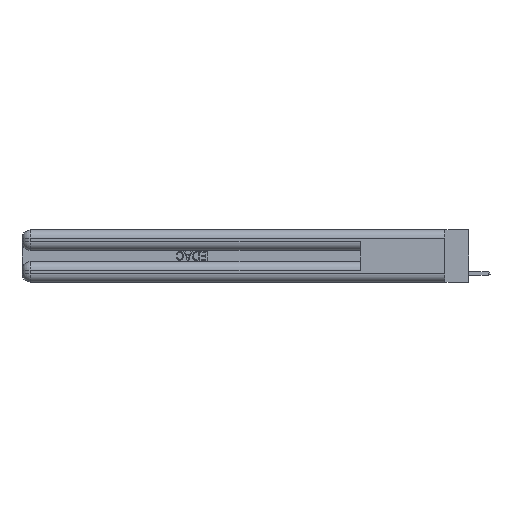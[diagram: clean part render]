
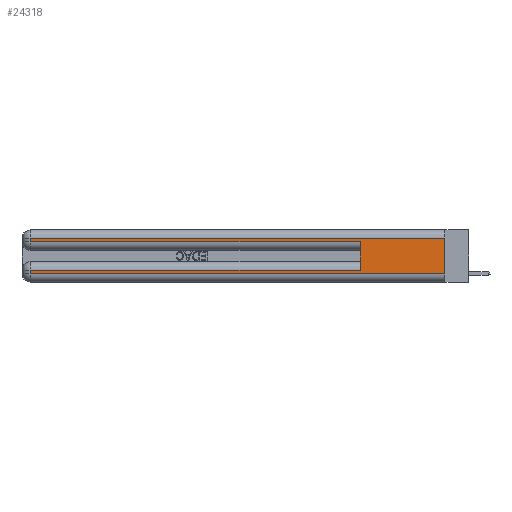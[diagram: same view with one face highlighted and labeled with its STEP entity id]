
A CAD part, left-side view. The second image highlights one B-rep face of the part: STEP entity #24318.
In plain terms, the highlighted planar face has unit normal (-1, 0, 0).
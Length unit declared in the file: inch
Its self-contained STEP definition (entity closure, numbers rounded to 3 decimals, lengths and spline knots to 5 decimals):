
#934 = DIRECTION ( 'NONE',  ( 0., 1., 0. ) ) ;
#1183 = DIRECTION ( 'NONE',  ( 0., -1., 0. ) ) ;
#1194 = VECTOR ( 'NONE', #3811, 39.37008 ) ;
#1406 = EDGE_LOOP ( 'NONE', ( #26395, #14939, #14035, #9605, #3924, #25589, #17612, #13681 ) ) ;
#1484 = EDGE_CURVE ( 'NONE', #33458, #34195, #20862, .T. ) ;
#1713 = VERTEX_POINT ( 'NONE', #23563 ) ;
#1804 = EDGE_CURVE ( 'NONE', #1713, #3582, #31366, .T. ) ;
#3386 = DIRECTION ( 'NONE',  ( 0., 0., -1. ) ) ;
#3582 = VERTEX_POINT ( 'NONE', #27402 ) ;
#3811 = DIRECTION ( 'NONE',  ( 0., 0., -1. ) ) ;
#3924 = ORIENTED_EDGE ( 'NONE', *, *, #13835, .F. ) ;
#4357 = CARTESIAN_POINT ( 'NONE',  ( 0., 2.94, 0.31 ) ) ;
#4922 = LINE ( 'NONE', #22695, #1194 ) ;
#5333 = VECTOR ( 'NONE', #3386, 39.37008 ) ;
#5536 = CARTESIAN_POINT ( 'NONE',  ( 0., 0.6, 0.145 ) ) ;
#5852 = CARTESIAN_POINT ( 'NONE',  ( 0., 0., 0.06 ) ) ;
#8537 = LINE ( 'NONE', #18350, #33734 ) ;
#8920 = CARTESIAN_POINT ( 'NONE',  ( 0., 0., 0.285 ) ) ;
#9605 = ORIENTED_EDGE ( 'NONE', *, *, #1484, .T. ) ;
#11579 = EDGE_CURVE ( 'NONE', #33373, #33458, #32306, .T. ) ;
#13681 = ORIENTED_EDGE ( 'NONE', *, *, #33790, .T. ) ;
#13835 = EDGE_CURVE ( 'NONE', #33293, #34195, #23214, .T. ) ;
#14035 = ORIENTED_EDGE ( 'NONE', *, *, #11579, .T. ) ;
#14939 = ORIENTED_EDGE ( 'NONE', *, *, #26741, .T. ) ;
#15154 = DIRECTION ( 'NONE',  ( 0., 1., 0. ) ) ;
#15432 = VECTOR ( 'NONE', #934, 39.37008 ) ;
#15842 = VECTOR ( 'NONE', #18857, 39.37008 ) ;
#16941 = CARTESIAN_POINT ( 'NONE',  ( 0., 2.94, 0.37 ) ) ;
#16946 = EDGE_CURVE ( 'NONE', #29055, #30956, #4922, .T. ) ;
#17269 = DIRECTION ( 'NONE',  ( 1., 0., 0. ) ) ;
#17492 = VECTOR ( 'NONE', #1183, 39.37008 ) ;
#17612 = ORIENTED_EDGE ( 'NONE', *, *, #1804, .T. ) ;
#18350 = CARTESIAN_POINT ( 'NONE',  ( 0., 0., 0.06 ) ) ;
#18857 = DIRECTION ( 'NONE',  ( 0., 0., -1. ) ) ;
#20640 = CARTESIAN_POINT ( 'NONE',  ( 0., 0.6, 0.085 ) ) ;
#20862 = LINE ( 'NONE', #8920, #17492 ) ;
#21330 = CARTESIAN_POINT ( 'NONE',  ( 0., 2.94, 0.37 ) ) ;
#22695 = CARTESIAN_POINT ( 'NONE',  ( 0., 0., 0.37 ) ) ;
#23214 = LINE ( 'NONE', #5536, #26163 ) ;
#23563 = CARTESIAN_POINT ( 'NONE',  ( 0., 2.94, 0.085 ) ) ;
#23775 = DIRECTION ( 'NONE',  ( 0., -1., 0. ) ) ;
#24248 = LINE ( 'NONE', #33930, #34741 ) ;
#24318 = ADVANCED_FACE ( 'NONE', ( #31562 ), #27409, .F. ) ;
#25128 = CARTESIAN_POINT ( 'NONE',  ( 0., 0., 0.085 ) ) ;
#25542 = DIRECTION ( 'NONE',  ( 0., 0., -1. ) ) ;
#25589 = ORIENTED_EDGE ( 'NONE', *, *, #26353, .T. ) ;
#26163 = VECTOR ( 'NONE', #32309, 39.37008 ) ;
#26353 = EDGE_CURVE ( 'NONE', #33293, #1713, #28062, .T. ) ;
#26395 = ORIENTED_EDGE ( 'NONE', *, *, #16946, .F. ) ;
#26723 = CARTESIAN_POINT ( 'NONE',  ( 0., 0., 0.31 ) ) ;
#26741 = EDGE_CURVE ( 'NONE', #29055, #33373, #24248, .T. ) ;
#27402 = CARTESIAN_POINT ( 'NONE',  ( 0., 2.94, 0.06 ) ) ;
#27409 = PLANE ( 'NONE',  #30368 ) ;
#28062 = LINE ( 'NONE', #25128, #15432 ) ;
#29055 = VERTEX_POINT ( 'NONE', #26723 ) ;
#30368 = AXIS2_PLACEMENT_3D ( 'NONE', #32815, #17269, #25542 ) ;
#30956 = VERTEX_POINT ( 'NONE', #5852 ) ;
#31366 = LINE ( 'NONE', #16941, #5333 ) ;
#31562 = FACE_OUTER_BOUND ( 'NONE', #1406, .T. ) ;
#32306 = LINE ( 'NONE', #21330, #15842 ) ;
#32309 = DIRECTION ( 'NONE',  ( 0., 0., 1. ) ) ;
#32815 = CARTESIAN_POINT ( 'NONE',  ( 0., 0., 0.37 ) ) ;
#33293 = VERTEX_POINT ( 'NONE', #20640 ) ;
#33373 = VERTEX_POINT ( 'NONE', #4357 ) ;
#33390 = CARTESIAN_POINT ( 'NONE',  ( 0., 0.6, 0.285 ) ) ;
#33458 = VERTEX_POINT ( 'NONE', #34629 ) ;
#33734 = VECTOR ( 'NONE', #23775, 39.37008 ) ;
#33790 = EDGE_CURVE ( 'NONE', #3582, #30956, #8537, .T. ) ;
#33930 = CARTESIAN_POINT ( 'NONE',  ( 0., 0., 0.31 ) ) ;
#34195 = VERTEX_POINT ( 'NONE', #33390 ) ;
#34629 = CARTESIAN_POINT ( 'NONE',  ( 0., 2.94, 0.285 ) ) ;
#34741 = VECTOR ( 'NONE', #15154, 39.37008 ) ;
